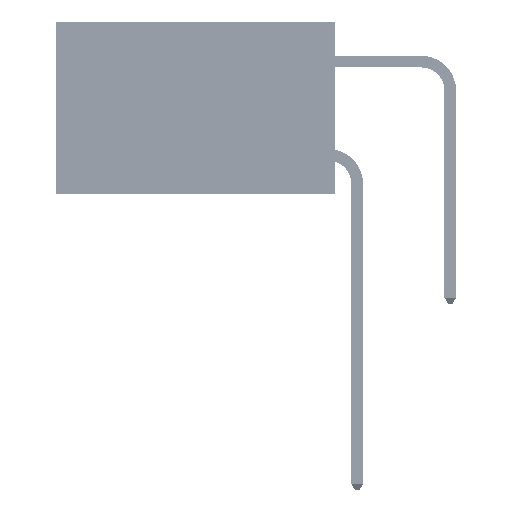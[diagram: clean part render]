
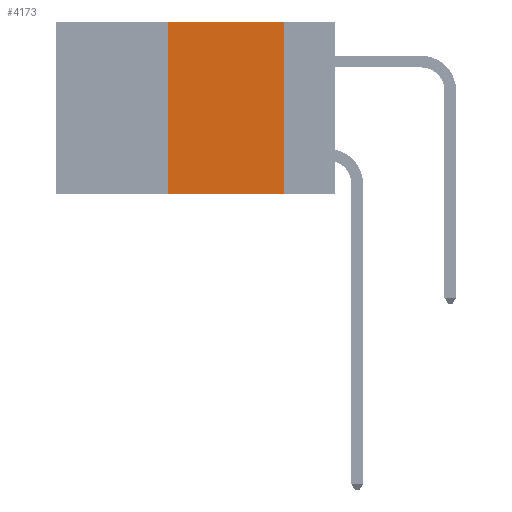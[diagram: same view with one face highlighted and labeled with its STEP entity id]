
A CAD part, left-side view. The second image highlights one B-rep face of the part: STEP entity #4173.
In plain terms, the highlighted planar face has unit normal (-1, 0, 0).
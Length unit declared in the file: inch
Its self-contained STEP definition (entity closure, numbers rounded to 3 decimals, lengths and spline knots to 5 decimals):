
#2558 = CARTESIAN_POINT ( 'NONE',  ( 0., 0.11, -0.37 ) ) ;
#2774 = ORIENTED_EDGE ( 'NONE', *, *, #20840, .F. ) ;
#3815 = CARTESIAN_POINT ( 'NONE',  ( 0., 0.36, 0. ) ) ;
#3985 = CARTESIAN_POINT ( 'NONE',  ( 0., 0.6, -0.37 ) ) ;
#4060 = LINE ( 'NONE', #45251, #24391 ) ;
#4173 = ADVANCED_FACE ( 'NONE', ( #6310 ), #43408, .F. ) ;
#4239 = CARTESIAN_POINT ( 'NONE',  ( 0., 0.6, 0. ) ) ;
#5163 = ORIENTED_EDGE ( 'NONE', *, *, #41997, .F. ) ;
#6310 = FACE_OUTER_BOUND ( 'NONE', #17210, .T. ) ;
#7676 = DIRECTION ( 'NONE',  ( 0., -1., 0. ) ) ;
#7777 = DIRECTION ( 'NONE',  ( 1., 0., 0. ) ) ;
#7904 = DIRECTION ( 'NONE',  ( 0., -1., 0. ) ) ;
#10239 = CARTESIAN_POINT ( 'NONE',  ( 0., 0.11, 0. ) ) ;
#15181 = CARTESIAN_POINT ( 'NONE',  ( 0., 0.36, -0.37 ) ) ;
#16611 = VECTOR ( 'NONE', #20746, 39.37008 ) ;
#17194 = CARTESIAN_POINT ( 'NONE',  ( 0., 0.11, 0. ) ) ;
#17210 = EDGE_LOOP ( 'NONE', ( #2774, #5163, #20996, #28379 ) ) ;
#17741 = LINE ( 'NONE', #17194, #16611 ) ;
#19742 = VECTOR ( 'NONE', #7676, 39.37008 ) ;
#20746 = DIRECTION ( 'NONE',  ( 0., 0., -1. ) ) ;
#20840 = EDGE_CURVE ( 'NONE', #36389, #43030, #17741, .T. ) ;
#20996 = ORIENTED_EDGE ( 'NONE', *, *, #42329, .F. ) ;
#24391 = VECTOR ( 'NONE', #27513, 39.37008 ) ;
#25646 = EDGE_CURVE ( 'NONE', #39172, #43030, #38705, .T. ) ;
#27200 = LINE ( 'NONE', #4239, #44994 ) ;
#27378 = AXIS2_PLACEMENT_3D ( 'NONE', #29236, #7777, #32788 ) ;
#27513 = DIRECTION ( 'NONE',  ( 0., 0., 1. ) ) ;
#28379 = ORIENTED_EDGE ( 'NONE', *, *, #25646, .T. ) ;
#29236 = CARTESIAN_POINT ( 'NONE',  ( 0., 0.6, 0. ) ) ;
#32788 = DIRECTION ( 'NONE',  ( 0., 0., -1. ) ) ;
#36389 = VERTEX_POINT ( 'NONE', #10239 ) ;
#36579 = VERTEX_POINT ( 'NONE', #3815 ) ;
#38705 = LINE ( 'NONE', #3985, #19742 ) ;
#39172 = VERTEX_POINT ( 'NONE', #15181 ) ;
#41997 = EDGE_CURVE ( 'NONE', #36579, #36389, #27200, .T. ) ;
#42329 = EDGE_CURVE ( 'NONE', #39172, #36579, #4060, .T. ) ;
#43030 = VERTEX_POINT ( 'NONE', #2558 ) ;
#43408 = PLANE ( 'NONE',  #27378 ) ;
#44994 = VECTOR ( 'NONE', #7904, 39.37008 ) ;
#45251 = CARTESIAN_POINT ( 'NONE',  ( 0., 0.36, 0. ) ) ;
